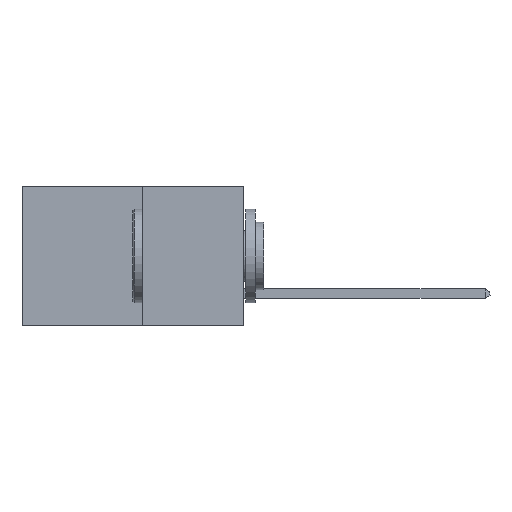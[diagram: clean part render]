
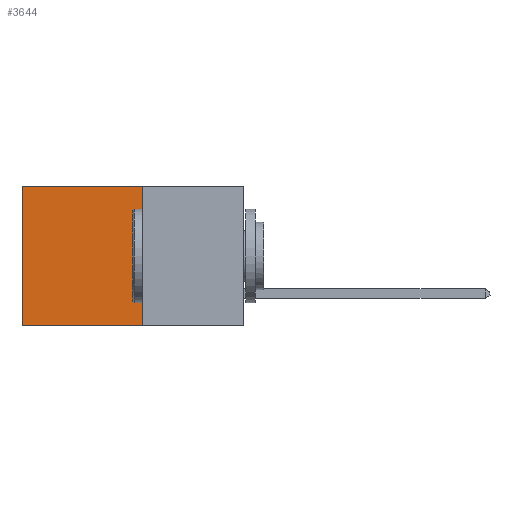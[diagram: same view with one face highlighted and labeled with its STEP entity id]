
A CAD part, left-side view. The second image highlights one B-rep face of the part: STEP entity #3644.
In plain terms, the highlighted planar face has unit normal (-1, 0, 0).
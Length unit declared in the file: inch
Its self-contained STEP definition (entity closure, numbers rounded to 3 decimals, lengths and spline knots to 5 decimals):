
#157 = AXIS2_PLACEMENT_3D ( 'NONE', #5211, #5164, #5139 ) ;
#359 = EDGE_CURVE ( 'NONE', #1899, #6731, #4746, .T. ) ;
#888 = CARTESIAN_POINT ( 'NONE',  ( 0.277, 0.27, -0.37 ) ) ;
#1094 = CARTESIAN_POINT ( 'NONE',  ( 0.277, 0.59, 0. ) ) ;
#1539 = CARTESIAN_POINT ( 'NONE',  ( 0.277, 0.59, -0.37 ) ) ;
#1899 = VERTEX_POINT ( 'NONE', #4355 ) ;
#1934 = VECTOR ( 'NONE', #6599, 39.37008 ) ;
#2666 = VERTEX_POINT ( 'NONE', #4898 ) ;
#3644 = ADVANCED_FACE ( 'NONE', ( #7613 ), #5219, .F. ) ;
#3971 = DIRECTION ( 'NONE',  ( 0., 1., 0. ) ) ;
#4025 = CARTESIAN_POINT ( 'NONE',  ( 0.277, 0.27, -0.37 ) ) ;
#4223 = VERTEX_POINT ( 'NONE', #1539 ) ;
#4355 = CARTESIAN_POINT ( 'NONE',  ( 0.277, 0.27, 0. ) ) ;
#4457 = ORIENTED_EDGE ( 'NONE', *, *, #4677, .F. ) ;
#4677 = EDGE_CURVE ( 'NONE', #2666, #4223, #11969, .T. ) ;
#4746 = LINE ( 'NONE', #10974, #9498 ) ;
#4898 = CARTESIAN_POINT ( 'NONE',  ( 0.277, 0.27, -0.37 ) ) ;
#4920 = ORIENTED_EDGE ( 'NONE', *, *, #359, .T. ) ;
#5139 = DIRECTION ( 'NONE',  ( 0., 0., -1. ) ) ;
#5164 = DIRECTION ( 'NONE',  ( 1., 0., 0. ) ) ;
#5211 = CARTESIAN_POINT ( 'NONE',  ( 0.277, 0.27, -0.37 ) ) ;
#5219 = PLANE ( 'NONE',  #157 ) ;
#5907 = VECTOR ( 'NONE', #6842, 39.37008 ) ;
#5945 = VECTOR ( 'NONE', #3971, 39.37008 ) ;
#6599 = DIRECTION ( 'NONE',  ( 0., 0., -1. ) ) ;
#6731 = VERTEX_POINT ( 'NONE', #1094 ) ;
#6842 = DIRECTION ( 'NONE',  ( 0., 0., -1. ) ) ;
#7438 = EDGE_LOOP ( 'NONE', ( #11422, #4457, #10178, #4920 ) ) ;
#7613 = FACE_OUTER_BOUND ( 'NONE', #7438, .T. ) ;
#8310 = DIRECTION ( 'NONE',  ( 0., 1., 0. ) ) ;
#8444 = LINE ( 'NONE', #888, #5907 ) ;
#8746 = EDGE_CURVE ( 'NONE', #6731, #4223, #11805, .T. ) ;
#8878 = EDGE_CURVE ( 'NONE', #1899, #2666, #8444, .T. ) ;
#9498 = VECTOR ( 'NONE', #8310, 39.37008 ) ;
#10178 = ORIENTED_EDGE ( 'NONE', *, *, #8878, .F. ) ;
#10974 = CARTESIAN_POINT ( 'NONE',  ( 0.277, 0.27, 0. ) ) ;
#11422 = ORIENTED_EDGE ( 'NONE', *, *, #8746, .T. ) ;
#11805 = LINE ( 'NONE', #12201, #1934 ) ;
#11969 = LINE ( 'NONE', #4025, #5945 ) ;
#12201 = CARTESIAN_POINT ( 'NONE',  ( 0.277, 0.59, -0.37 ) ) ;
